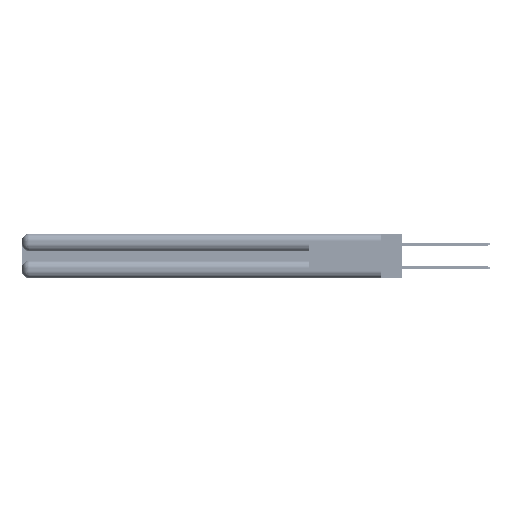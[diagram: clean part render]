
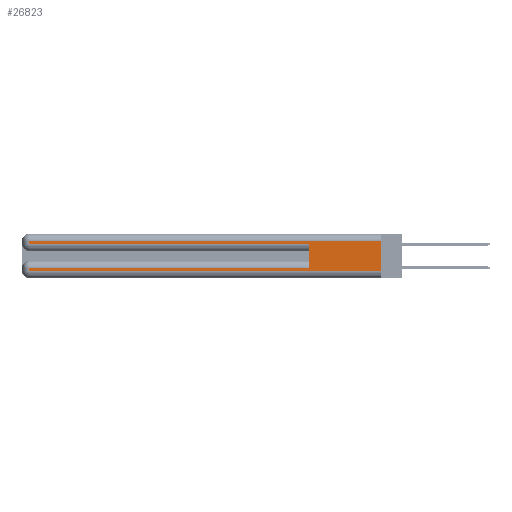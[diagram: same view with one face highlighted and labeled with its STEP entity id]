
A CAD part, left-side view. The second image highlights one B-rep face of the part: STEP entity #26823.
In plain terms, the highlighted planar face has unit normal (-1, 0, 0).
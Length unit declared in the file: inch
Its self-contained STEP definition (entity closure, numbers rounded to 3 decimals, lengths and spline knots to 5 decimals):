
#501 = DIRECTION ( 'NONE',  ( 0., 0., -1. ) ) ;
#1394 = LINE ( 'NONE', #47219, #21922 ) ;
#2299 = LINE ( 'NONE', #33794, #45539 ) ;
#3709 = VECTOR ( 'NONE', #26721, 39.37008 ) ;
#3929 = CARTESIAN_POINT ( 'NONE',  ( 0., 0.6, 0.085 ) ) ;
#4179 = ORIENTED_EDGE ( 'NONE', *, *, #16277, .F. ) ;
#4331 = VERTEX_POINT ( 'NONE', #9787 ) ;
#5234 = ORIENTED_EDGE ( 'NONE', *, *, #10077, .T. ) ;
#5487 = CARTESIAN_POINT ( 'NONE',  ( 0., 0.6, 0.285 ) ) ;
#5667 = DIRECTION ( 'NONE',  ( 0., -1., 0. ) ) ;
#5882 = EDGE_CURVE ( 'NONE', #18103, #43334, #39321, .T. ) ;
#6022 = VECTOR ( 'NONE', #5667, 39.37008 ) ;
#6905 = VECTOR ( 'NONE', #11692, 39.37008 ) ;
#7864 = VECTOR ( 'NONE', #501, 39.37008 ) ;
#8907 = AXIS2_PLACEMENT_3D ( 'NONE', #10535, #18718, #46984 ) ;
#9435 = DIRECTION ( 'NONE',  ( 0., 0., -1. ) ) ;
#9787 = CARTESIAN_POINT ( 'NONE',  ( 0., 2.94, 0.31 ) ) ;
#10077 = EDGE_CURVE ( 'NONE', #51174, #34508, #22924, .T. ) ;
#10535 = CARTESIAN_POINT ( 'NONE',  ( 0., 0., 0.37 ) ) ;
#11692 = DIRECTION ( 'NONE',  ( 0., -1., 0. ) ) ;
#12594 = VECTOR ( 'NONE', #27073, 39.37008 ) ;
#14097 = LINE ( 'NONE', #50860, #3709 ) ;
#14615 = CARTESIAN_POINT ( 'NONE',  ( 0., 0., 0.31 ) ) ;
#14661 = PLANE ( 'NONE',  #8907 ) ;
#16277 = EDGE_CURVE ( 'NONE', #24414, #27200, #30790, .T. ) ;
#16289 = ORIENTED_EDGE ( 'NONE', *, *, #18636, .T. ) ;
#18103 = VERTEX_POINT ( 'NONE', #51595 ) ;
#18636 = EDGE_CURVE ( 'NONE', #24414, #4331, #14097, .T. ) ;
#18718 = DIRECTION ( 'NONE',  ( 1., 0., 0. ) ) ;
#20192 = CARTESIAN_POINT ( 'NONE',  ( 0., 2.94, 0.085 ) ) ;
#21327 = DIRECTION ( 'NONE',  ( 0., 0., -1. ) ) ;
#21719 = ORIENTED_EDGE ( 'NONE', *, *, #47282, .T. ) ;
#21922 = VECTOR ( 'NONE', #31200, 39.37008 ) ;
#22924 = LINE ( 'NONE', #33355, #32412 ) ;
#23012 = CARTESIAN_POINT ( 'NONE',  ( 0., 0.6, 0.145 ) ) ;
#23471 = VERTEX_POINT ( 'NONE', #3929 ) ;
#24166 = ORIENTED_EDGE ( 'NONE', *, *, #41366, .T. ) ;
#24414 = VERTEX_POINT ( 'NONE', #14615 ) ;
#26721 = DIRECTION ( 'NONE',  ( 0., 1., 0. ) ) ;
#26823 = ADVANCED_FACE ( 'NONE', ( #33989 ), #14661, .F. ) ;
#27073 = DIRECTION ( 'NONE',  ( 0., 0., 1. ) ) ;
#27200 = VERTEX_POINT ( 'NONE', #37297 ) ;
#27740 = LINE ( 'NONE', #34167, #6022 ) ;
#27899 = CARTESIAN_POINT ( 'NONE',  ( 0., 0., 0.285 ) ) ;
#29523 = CARTESIAN_POINT ( 'NONE',  ( 0., 2.94, 0.06 ) ) ;
#30790 = LINE ( 'NONE', #33182, #7864 ) ;
#31200 = DIRECTION ( 'NONE',  ( 0., 1., 0. ) ) ;
#32412 = VECTOR ( 'NONE', #21327, 39.37008 ) ;
#33182 = CARTESIAN_POINT ( 'NONE',  ( 0., 0., 0.37 ) ) ;
#33355 = CARTESIAN_POINT ( 'NONE',  ( 0., 2.94, 0.37 ) ) ;
#33794 = CARTESIAN_POINT ( 'NONE',  ( 0., 2.94, 0.37 ) ) ;
#33989 = FACE_OUTER_BOUND ( 'NONE', #45541, .T. ) ;
#34167 = CARTESIAN_POINT ( 'NONE',  ( 0., 0., 0.06 ) ) ;
#34508 = VERTEX_POINT ( 'NONE', #29523 ) ;
#37297 = CARTESIAN_POINT ( 'NONE',  ( 0., 0., 0.06 ) ) ;
#38845 = EDGE_CURVE ( 'NONE', #34508, #27200, #27740, .T. ) ;
#39321 = LINE ( 'NONE', #27899, #6905 ) ;
#39836 = ORIENTED_EDGE ( 'NONE', *, *, #38845, .T. ) ;
#41366 = EDGE_CURVE ( 'NONE', #4331, #18103, #2299, .T. ) ;
#41619 = EDGE_CURVE ( 'NONE', #23471, #43334, #44876, .T. ) ;
#43113 = ORIENTED_EDGE ( 'NONE', *, *, #41619, .F. ) ;
#43334 = VERTEX_POINT ( 'NONE', #5487 ) ;
#44876 = LINE ( 'NONE', #23012, #12594 ) ;
#45539 = VECTOR ( 'NONE', #9435, 39.37008 ) ;
#45541 = EDGE_LOOP ( 'NONE', ( #4179, #16289, #24166, #45592, #43113, #21719, #5234, #39836 ) ) ;
#45592 = ORIENTED_EDGE ( 'NONE', *, *, #5882, .T. ) ;
#46984 = DIRECTION ( 'NONE',  ( 0., 0., -1. ) ) ;
#47219 = CARTESIAN_POINT ( 'NONE',  ( 0., 0., 0.085 ) ) ;
#47282 = EDGE_CURVE ( 'NONE', #23471, #51174, #1394, .T. ) ;
#50860 = CARTESIAN_POINT ( 'NONE',  ( 0., 0., 0.31 ) ) ;
#51174 = VERTEX_POINT ( 'NONE', #20192 ) ;
#51595 = CARTESIAN_POINT ( 'NONE',  ( 0., 2.94, 0.285 ) ) ;
